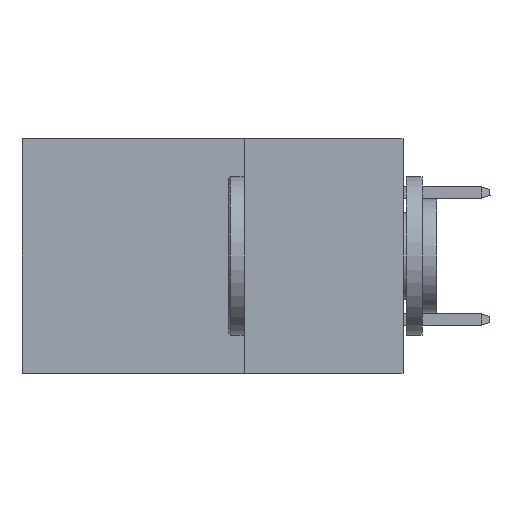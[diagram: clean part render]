
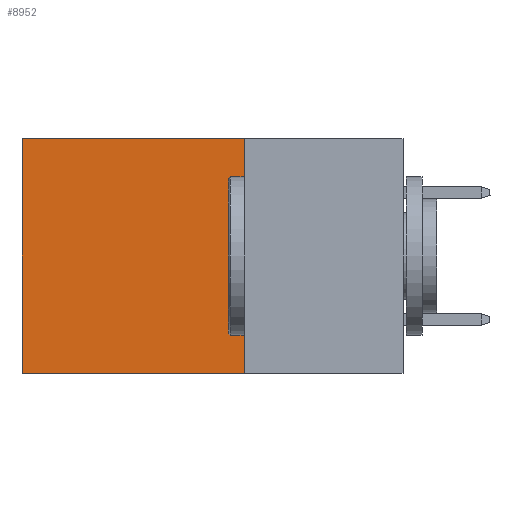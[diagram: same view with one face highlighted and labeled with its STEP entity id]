
A CAD part, left-side view. The second image highlights one B-rep face of the part: STEP entity #8952.
In plain terms, the highlighted planar face has unit normal (-1, 0, 0).
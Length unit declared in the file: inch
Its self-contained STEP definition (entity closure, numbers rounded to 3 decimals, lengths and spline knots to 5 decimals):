
#1679 = LINE ( 'NONE', #42560, #40562 ) ;
#2325 = EDGE_CURVE ( 'NONE', #32387, #32782, #1679, .T. ) ;
#2951 = EDGE_CURVE ( 'NONE', #30857, #27338, #41517, .T. ) ;
#3130 = DIRECTION ( 'NONE',  ( 0., 0., -1. ) ) ;
#3982 = AXIS2_PLACEMENT_3D ( 'NONE', #8807, #12604, #32710 ) ;
#4296 = ORIENTED_EDGE ( 'NONE', *, *, #2325, .F. ) ;
#7435 = LINE ( 'NONE', #16488, #15381 ) ;
#7795 = DIRECTION ( 'NONE',  ( 0., 1., 0. ) ) ;
#8104 = ORIENTED_EDGE ( 'NONE', *, *, #2951, .T. ) ;
#8807 = CARTESIAN_POINT ( 'NONE',  ( 0.2875, 0.25, 0. ) ) ;
#8952 = ADVANCED_FACE ( 'NONE', ( #33127 ), #19522, .F. ) ;
#10729 = CARTESIAN_POINT ( 'NONE',  ( 0.2875, 0.25, 0. ) ) ;
#12604 = DIRECTION ( 'NONE',  ( 1., 0., 0. ) ) ;
#15381 = VECTOR ( 'NONE', #41393, 39.37008 ) ;
#16488 = CARTESIAN_POINT ( 'NONE',  ( 0.2875, 0.6, 0. ) ) ;
#19522 = PLANE ( 'NONE',  #3982 ) ;
#20344 = LINE ( 'NONE', #10729, #42904 ) ;
#20768 = CARTESIAN_POINT ( 'NONE',  ( 0.2875, 0.25, 0. ) ) ;
#21885 = CARTESIAN_POINT ( 'NONE',  ( 0.2875, 0.6, -0.37 ) ) ;
#23122 = DIRECTION ( 'NONE',  ( 0., 1., 0. ) ) ;
#23732 = CARTESIAN_POINT ( 'NONE',  ( 0.2875, 0.6, 0. ) ) ;
#27338 = VERTEX_POINT ( 'NONE', #23732 ) ;
#28270 = EDGE_LOOP ( 'NONE', ( #32479, #4296, #39479, #8104 ) ) ;
#28400 = CARTESIAN_POINT ( 'NONE',  ( 0.2875, 0.25, 0. ) ) ;
#30264 = EDGE_CURVE ( 'NONE', #27338, #32782, #7435, .T. ) ;
#30857 = VERTEX_POINT ( 'NONE', #28400 ) ;
#32387 = VERTEX_POINT ( 'NONE', #41401 ) ;
#32479 = ORIENTED_EDGE ( 'NONE', *, *, #30264, .T. ) ;
#32710 = DIRECTION ( 'NONE',  ( 0., 0., -1. ) ) ;
#32782 = VERTEX_POINT ( 'NONE', #21885 ) ;
#33127 = FACE_OUTER_BOUND ( 'NONE', #28270, .T. ) ;
#36317 = VECTOR ( 'NONE', #7795, 39.37008 ) ;
#36442 = EDGE_CURVE ( 'NONE', #30857, #32387, #20344, .T. ) ;
#39479 = ORIENTED_EDGE ( 'NONE', *, *, #36442, .F. ) ;
#40562 = VECTOR ( 'NONE', #23122, 39.37008 ) ;
#41393 = DIRECTION ( 'NONE',  ( 0., 0., -1. ) ) ;
#41401 = CARTESIAN_POINT ( 'NONE',  ( 0.2875, 0.25, -0.37 ) ) ;
#41517 = LINE ( 'NONE', #20768, #36317 ) ;
#42560 = CARTESIAN_POINT ( 'NONE',  ( 0.2875, 0.25, -0.37 ) ) ;
#42904 = VECTOR ( 'NONE', #3130, 39.37008 ) ;
